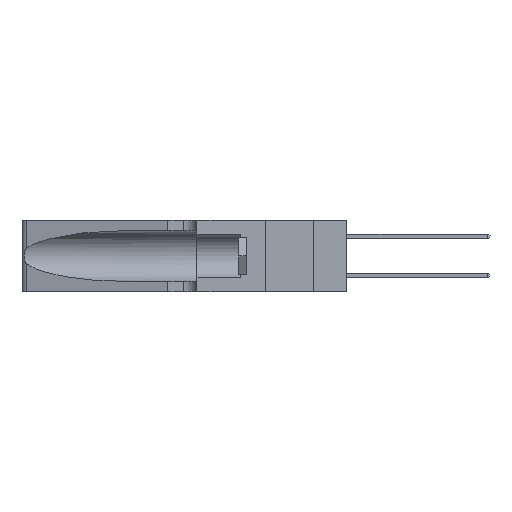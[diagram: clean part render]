
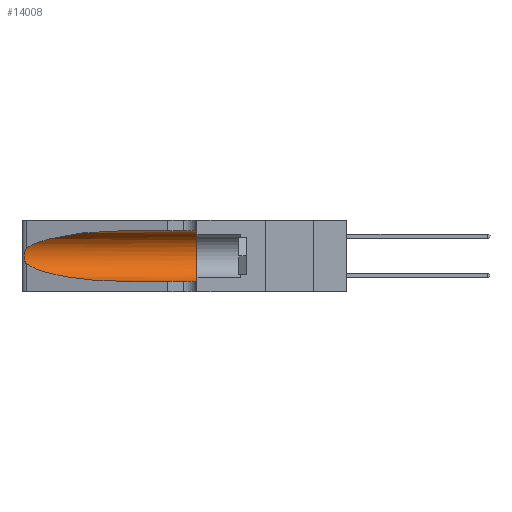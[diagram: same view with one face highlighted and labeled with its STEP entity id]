
A CAD part, left-side view. The second image highlights one B-rep face of the part: STEP entity #14008.
In plain terms, the highlighted cylindrical face has radius 3.308 mm (diameter 6.617 mm), a partial arc.
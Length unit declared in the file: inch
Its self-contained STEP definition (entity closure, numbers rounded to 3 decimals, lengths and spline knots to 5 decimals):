
#964 = EDGE_LOOP ( 'NONE', ( #30241, #1934, #5994, #7143, #8023, #40202 ) ) ;
#1355 = DIRECTION ( 'NONE',  ( 0., -1., 0. ) ) ;
#1934 = ORIENTED_EDGE ( 'NONE', *, *, #15301, .T. ) ;
#2407 = LINE ( 'NONE', #18967, #11343 ) ;
#4186 = EDGE_CURVE ( 'NONE', #28806, #45727, #23313, .T. ) ;
#5083 = CARTESIAN_POINT ( 'NONE',  ( 0.1305, 1.61858, 0.31525 ) ) ;
#5116 = LINE ( 'NONE', #5083, #7913 ) ;
#5778 = CARTESIAN_POINT ( 'NONE',  ( 0.25854, 1.2359, 0.20912 ) ) ;
#5994 = ORIENTED_EDGE ( 'NONE', *, *, #41015, .T. ) ;
#6243 = CARTESIAN_POINT ( 'NONE',  ( 0.25639, 1.23184, 0.21858 ) ) ;
#6401 = CARTESIAN_POINT ( 'NONE',  ( 0.25555, 1.22994, 0.2215 ) ) ;
#7143 = ORIENTED_EDGE ( 'NONE', *, *, #39525, .T. ) ;
#7590 = CARTESIAN_POINT ( 'NONE',  ( 0.2373, 1.15595, 0.28018 ) ) ;
#7913 = VECTOR ( 'NONE', #26868, 39.37008 ) ;
#8023 = ORIENTED_EDGE ( 'NONE', *, *, #4186, .F. ) ;
#8666 = CARTESIAN_POINT ( 'NONE',  ( 0.1305, 0.35, 0.05475 ) ) ;
#9492 = EDGE_CURVE ( 'NONE', #26365, #44753, #18177, .T. ) ;
#9702 = CARTESIAN_POINT ( 'NONE',  ( 0.25856, 1.23593, 0.16098 ) ) ;
#9850 = CARTESIAN_POINT ( 'NONE',  ( 0.25555, 1.22993, 0.14849 ) ) ;
#10105 = CARTESIAN_POINT ( 'NONE',  ( 0.18966, 0.96281, 0.31525 ) ) ;
#11196 = EDGE_CURVE ( 'NONE', #26365, #28806, #5116, .T. ) ;
#11343 = VECTOR ( 'NONE', #1355, 39.37008 ) ;
#12022 = VERTEX_POINT ( 'NONE', #17601 ) ;
#12140 = CARTESIAN_POINT ( 'NONE',  ( 0.1305, 0.35, 0.31525 ) ) ;
#12682 = DIRECTION ( 'NONE',  ( 0., 0., 1. ) ) ;
#14008 = ADVANCED_FACE ( 'NONE', ( #18580 ), #38121, .F. ) ;
#15301 = EDGE_CURVE ( 'NONE', #44753, #12022, #15336, .T. ) ;
#15336 = B_SPLINE_CURVE_WITH_KNOTS ( 'NONE', 3,
 ( #41406, #6401, #6243, #31163, #5778, #20401, #34745, #41714, #38316, #9702, #16351, #45144, #9850, #45286 ),
 .UNSPECIFIED., .F., .F.,
 ( 4, 2, 2, 2, 2, 2, 4 ),
 ( 0., 0.00027, 0.00053, 0.00107, 0.0016, 0.00187, 0.00214 ),
 .UNSPECIFIED. ) ;
#16351 = CARTESIAN_POINT ( 'NONE',  ( 0.25789, 1.23486, 0.15765 ) ) ;
#16495 = CARTESIAN_POINT ( 'NONE',  ( 0.1305, 0.72297, 0.05475 ) ) ;
#17601 = CARTESIAN_POINT ( 'NONE',  ( 0.25487, 1.22718, 0.14631 ) ) ;
#18177 =( BOUNDED_CURVE ( )  B_SPLINE_CURVE ( 3, ( #24221, #10105, #7590, #34988 ),
 .UNSPECIFIED., .F., .T. ) 
 B_SPLINE_CURVE_WITH_KNOTS ( ( 4, 4 ),
 ( 1.5708, 2.84003 ),
 .UNSPECIFIED. ) 
 CURVE ( )  GEOMETRIC_REPRESENTATION_ITEM ( )  RATIONAL_B_SPLINE_CURVE ( ( 1., 0.87, 0.87, 1. ) ) 
 REPRESENTATION_ITEM ( '' )  );
#18580 = FACE_OUTER_BOUND ( 'NONE', #964, .T. ) ;
#18967 = CARTESIAN_POINT ( 'NONE',  ( 0.1305, 1.61858, 0.05475 ) ) ;
#19911 = CARTESIAN_POINT ( 'NONE',  ( 0.1305, 1.61858, 0.185 ) ) ;
#20401 = CARTESIAN_POINT ( 'NONE',  ( 0.26018, 1.23835, 0.19895 ) ) ;
#23313 = CIRCLE ( 'NONE', #27184, 0.13025 ) ;
#23868 = DIRECTION ( 'NONE',  ( 0., 1., 0. ) ) ;
#24221 = CARTESIAN_POINT ( 'NONE',  ( 0.1305, 0.72297, 0.31525 ) ) ;
#25876 = VERTEX_POINT ( 'NONE', #38539 ) ;
#26365 = VERTEX_POINT ( 'NONE', #31011 ) ;
#26868 = DIRECTION ( 'NONE',  ( 0., -1., 0. ) ) ;
#27142 = CARTESIAN_POINT ( 'NONE',  ( 0.1305, 0.35, 0.185 ) ) ;
#27184 = AXIS2_PLACEMENT_3D ( 'NONE', #27142, #23868, #12682 ) ;
#28039 = CARTESIAN_POINT ( 'NONE',  ( 0.25487, 1.22718, 0.22369 ) ) ;
#28737 =( BOUNDED_CURVE ( )  B_SPLINE_CURVE ( 3, ( #34435, #34588, #34124, #16495 ),
 .UNSPECIFIED., .F., .F. ) 
 B_SPLINE_CURVE_WITH_KNOTS ( ( 4, 4 ),
 ( 3.44316, 4.71239 ),
 .UNSPECIFIED. ) 
 CURVE ( )  GEOMETRIC_REPRESENTATION_ITEM ( )  RATIONAL_B_SPLINE_CURVE ( ( 1., 0.87, 0.87, 1. ) ) 
 REPRESENTATION_ITEM ( '' )  );
#28806 = VERTEX_POINT ( 'NONE', #12140 ) ;
#30241 = ORIENTED_EDGE ( 'NONE', *, *, #9492, .T. ) ;
#30808 = DIRECTION ( 'NONE',  ( 0., 0., -1. ) ) ;
#31011 = CARTESIAN_POINT ( 'NONE',  ( 0.1305, 0.72297, 0.31525 ) ) ;
#31163 = CARTESIAN_POINT ( 'NONE',  ( 0.25787, 1.23484, 0.2124 ) ) ;
#34124 = CARTESIAN_POINT ( 'NONE',  ( 0.18966, 0.96281, 0.05475 ) ) ;
#34435 = CARTESIAN_POINT ( 'NONE',  ( 0.25487, 1.22718, 0.14631 ) ) ;
#34588 = CARTESIAN_POINT ( 'NONE',  ( 0.2373, 1.15595, 0.08982 ) ) ;
#34745 = CARTESIAN_POINT ( 'NONE',  ( 0.26075, 1.23896, 0.19203 ) ) ;
#34988 = CARTESIAN_POINT ( 'NONE',  ( 0.25487, 1.22718, 0.22369 ) ) ;
#38121 = CYLINDRICAL_SURFACE ( 'NONE', #38742, 0.13025 ) ;
#38316 = CARTESIAN_POINT ( 'NONE',  ( 0.26017, 1.23833, 0.17102 ) ) ;
#38539 = CARTESIAN_POINT ( 'NONE',  ( 0.1305, 0.72297, 0.05475 ) ) ;
#38742 = AXIS2_PLACEMENT_3D ( 'NONE', #19911, #44484, #30808 ) ;
#39525 = EDGE_CURVE ( 'NONE', #25876, #45727, #2407, .T. ) ;
#40202 = ORIENTED_EDGE ( 'NONE', *, *, #11196, .F. ) ;
#41015 = EDGE_CURVE ( 'NONE', #12022, #25876, #28737, .T. ) ;
#41406 = CARTESIAN_POINT ( 'NONE',  ( 0.25487, 1.22718, 0.22369 ) ) ;
#41714 = CARTESIAN_POINT ( 'NONE',  ( 0.26075, 1.23896, 0.178 ) ) ;
#44484 = DIRECTION ( 'NONE',  ( 0., -1., 0. ) ) ;
#44753 = VERTEX_POINT ( 'NONE', #28039 ) ;
#45144 = CARTESIAN_POINT ( 'NONE',  ( 0.25639, 1.23186, 0.15144 ) ) ;
#45286 = CARTESIAN_POINT ( 'NONE',  ( 0.25487, 1.22718, 0.14631 ) ) ;
#45727 = VERTEX_POINT ( 'NONE', #8666 ) ;
